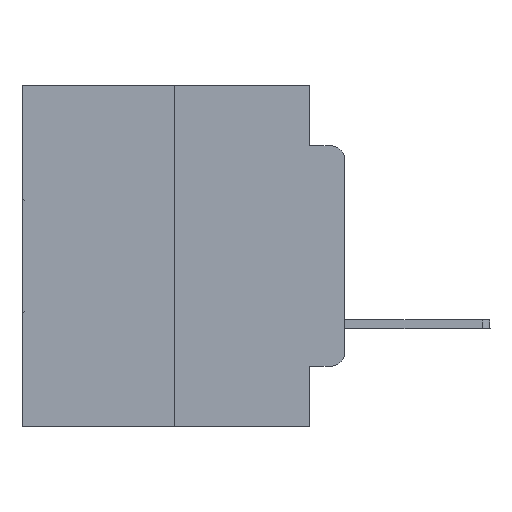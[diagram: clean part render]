
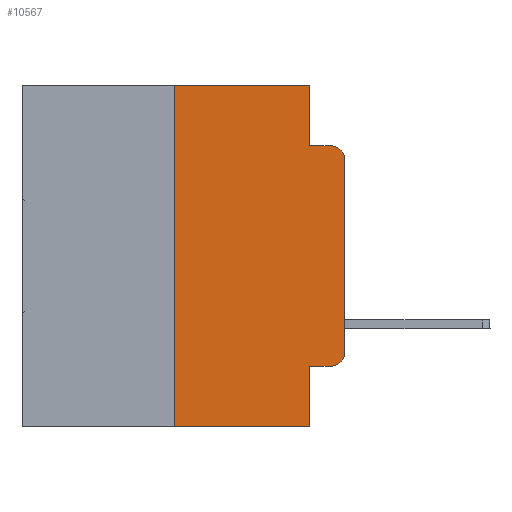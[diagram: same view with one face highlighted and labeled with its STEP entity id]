
A CAD part, left-side view. The second image highlights one B-rep face of the part: STEP entity #10567.
In plain terms, the highlighted planar face has unit normal (-1, 0, 0).
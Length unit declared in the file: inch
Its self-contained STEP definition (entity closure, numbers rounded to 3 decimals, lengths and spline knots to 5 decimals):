
#552 = VERTEX_POINT ( 'NONE', #6743 ) ;
#595 = CARTESIAN_POINT ( 'NONE',  ( 0., 0., -0.3915 ) ) ;
#602 = DIRECTION ( 'NONE',  ( -1., 0., 0. ) ) ;
#640 = ORIENTED_EDGE ( 'NONE', *, *, #14991, .T. ) ;
#941 = DIRECTION ( 'NONE',  ( 0., 0., -1. ) ) ;
#1054 = LINE ( 'NONE', #28589, #11300 ) ;
#1063 = DIRECTION ( 'NONE',  ( 1., 0., 0. ) ) ;
#1275 = DIRECTION ( 'NONE',  ( 0., 0., -1. ) ) ;
#1516 = EDGE_LOOP ( 'NONE', ( #12615, #23608, #11350, #10824, #6260, #14453, #14666, #26077, #9543, #640 ) ) ;
#2248 = EDGE_CURVE ( 'NONE', #23223, #8260, #15045, .T. ) ;
#2875 = LINE ( 'NONE', #23308, #23299 ) ;
#3278 = CARTESIAN_POINT ( 'NONE',  ( 0., 0.051, -0.4115 ) ) ;
#3765 = LINE ( 'NONE', #16890, #4810 ) ;
#4135 = VERTEX_POINT ( 'NONE', #7620 ) ;
#4810 = VECTOR ( 'NONE', #1275, 39.37008 ) ;
#4892 = DIRECTION ( 'NONE',  ( 0., -1., 0. ) ) ;
#4926 = CARTESIAN_POINT ( 'NONE',  ( 0., 0.473, 0. ) ) ;
#4985 = DIRECTION ( 'NONE',  ( 0., -1., 0. ) ) ;
#5209 = LINE ( 'NONE', #18257, #21766 ) ;
#5219 = VERTEX_POINT ( 'NONE', #3278 ) ;
#6260 = ORIENTED_EDGE ( 'NONE', *, *, #15036, .F. ) ;
#6743 = CARTESIAN_POINT ( 'NONE',  ( 0., 0., -0.1085 ) ) ;
#7154 = DIRECTION ( 'NONE',  ( 0., 0., -1. ) ) ;
#7620 = CARTESIAN_POINT ( 'NONE',  ( 0., 0.051, -0.5 ) ) ;
#7663 = VECTOR ( 'NONE', #12652, 39.37008 ) ;
#7667 = EDGE_CURVE ( 'NONE', #25462, #28437, #3765, .T. ) ;
#8260 = VERTEX_POINT ( 'NONE', #9359 ) ;
#9359 = CARTESIAN_POINT ( 'NONE',  ( 0., 0.25, 0. ) ) ;
#9475 = DIRECTION ( 'NONE',  ( 0., -1., 0. ) ) ;
#9543 = ORIENTED_EDGE ( 'NONE', *, *, #14375, .T. ) ;
#9573 = LINE ( 'NONE', #18353, #26433 ) ;
#10193 = AXIS2_PLACEMENT_3D ( 'NONE', #11824, #602, #20667 ) ;
#10567 = ADVANCED_FACE ( 'NONE', ( #28280 ), #14406, .F. ) ;
#10824 = ORIENTED_EDGE ( 'NONE', *, *, #7667, .F. ) ;
#11300 = VECTOR ( 'NONE', #15025, 39.37008 ) ;
#11350 = ORIENTED_EDGE ( 'NONE', *, *, #16216, .F. ) ;
#11365 = CARTESIAN_POINT ( 'NONE',  ( 0., 0.25, -0.5 ) ) ;
#11561 = EDGE_CURVE ( 'NONE', #552, #28073, #19602, .T. ) ;
#11616 = AXIS2_PLACEMENT_3D ( 'NONE', #14515, #1063, #16765 ) ;
#11824 = CARTESIAN_POINT ( 'NONE',  ( 0., 0.02, -0.3915 ) ) ;
#12140 = DIRECTION ( 'NONE',  ( -1., 0., 0. ) ) ;
#12615 = ORIENTED_EDGE ( 'NONE', *, *, #20078, .T. ) ;
#12652 = DIRECTION ( 'NONE',  ( 0., 0., 1. ) ) ;
#14348 = DIRECTION ( 'NONE',  ( 0., 0., 1. ) ) ;
#14375 = EDGE_CURVE ( 'NONE', #5219, #25528, #23677, .T. ) ;
#14406 = PLANE ( 'NONE',  #11616 ) ;
#14453 = ORIENTED_EDGE ( 'NONE', *, *, #2248, .F. ) ;
#14515 = CARTESIAN_POINT ( 'NONE',  ( 0., 0.473, 0. ) ) ;
#14666 = ORIENTED_EDGE ( 'NONE', *, *, #21967, .T. ) ;
#14799 = CARTESIAN_POINT ( 'NONE',  ( 0., 0.25, 0. ) ) ;
#14991 = EDGE_CURVE ( 'NONE', #25528, #23295, #25357, .T. ) ;
#15025 = DIRECTION ( 'NONE',  ( 0., -1., 0. ) ) ;
#15036 = EDGE_CURVE ( 'NONE', #8260, #25462, #18679, .T. ) ;
#15045 = LINE ( 'NONE', #14799, #7663 ) ;
#15117 = EDGE_CURVE ( 'NONE', #5219, #4135, #9573, .T. ) ;
#15601 = CARTESIAN_POINT ( 'NONE',  ( 0., 0.02, -0.4115 ) ) ;
#16216 = EDGE_CURVE ( 'NONE', #28437, #28073, #1054, .T. ) ;
#16765 = DIRECTION ( 'NONE',  ( 0., 0., -1. ) ) ;
#16890 = CARTESIAN_POINT ( 'NONE',  ( 0., 0.051, 0. ) ) ;
#17305 = CARTESIAN_POINT ( 'NONE',  ( 0., 0.051, 0. ) ) ;
#18257 = CARTESIAN_POINT ( 'NONE',  ( 0., 0.473, -0.5 ) ) ;
#18353 = CARTESIAN_POINT ( 'NONE',  ( 0., 0.051, 0. ) ) ;
#18361 = CARTESIAN_POINT ( 'NONE',  ( 0., 0.051, -0.4115 ) ) ;
#18679 = LINE ( 'NONE', #4926, #22234 ) ;
#19602 = CIRCLE ( 'NONE', #20861, 0.02 ) ;
#20078 = EDGE_CURVE ( 'NONE', #23295, #552, #2875, .T. ) ;
#20503 = VECTOR ( 'NONE', #4892, 39.37008 ) ;
#20667 = DIRECTION ( 'NONE',  ( 0., 0., -1. ) ) ;
#20861 = AXIS2_PLACEMENT_3D ( 'NONE', #21391, #12140, #941 ) ;
#21391 = CARTESIAN_POINT ( 'NONE',  ( 0., 0.02, -0.1085 ) ) ;
#21766 = VECTOR ( 'NONE', #4985, 39.37008 ) ;
#21967 = EDGE_CURVE ( 'NONE', #23223, #4135, #5209, .T. ) ;
#22234 = VECTOR ( 'NONE', #9475, 39.37008 ) ;
#23060 = CARTESIAN_POINT ( 'NONE',  ( 0., 0.02, -0.0885 ) ) ;
#23223 = VERTEX_POINT ( 'NONE', #11365 ) ;
#23295 = VERTEX_POINT ( 'NONE', #595 ) ;
#23299 = VECTOR ( 'NONE', #14348, 39.37008 ) ;
#23308 = CARTESIAN_POINT ( 'NONE',  ( 0., 0., 0. ) ) ;
#23608 = ORIENTED_EDGE ( 'NONE', *, *, #11561, .T. ) ;
#23677 = LINE ( 'NONE', #18361, #20503 ) ;
#25357 = CIRCLE ( 'NONE', #10193, 0.02 ) ;
#25462 = VERTEX_POINT ( 'NONE', #17305 ) ;
#25528 = VERTEX_POINT ( 'NONE', #15601 ) ;
#26077 = ORIENTED_EDGE ( 'NONE', *, *, #15117, .F. ) ;
#26433 = VECTOR ( 'NONE', #7154, 39.37008 ) ;
#26582 = CARTESIAN_POINT ( 'NONE',  ( 0., 0.051, -0.0885 ) ) ;
#28073 = VERTEX_POINT ( 'NONE', #23060 ) ;
#28280 = FACE_OUTER_BOUND ( 'NONE', #1516, .T. ) ;
#28437 = VERTEX_POINT ( 'NONE', #26582 ) ;
#28589 = CARTESIAN_POINT ( 'NONE',  ( 0., 0.051, -0.0885 ) ) ;
